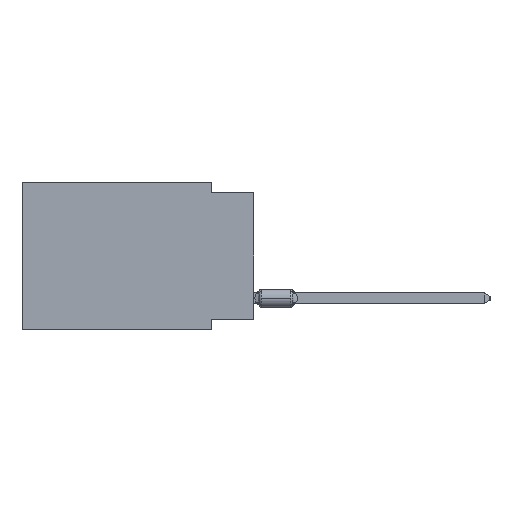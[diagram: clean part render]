
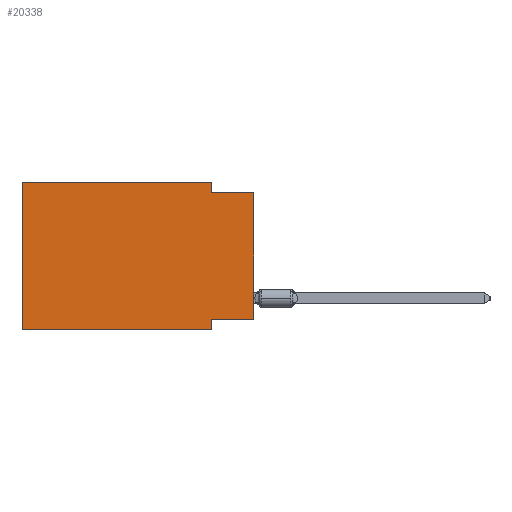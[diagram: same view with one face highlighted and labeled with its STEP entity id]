
A CAD part, left-side view. The second image highlights one B-rep face of the part: STEP entity #20338.
In plain terms, the highlighted planar face has unit normal (-1, 0, 0).
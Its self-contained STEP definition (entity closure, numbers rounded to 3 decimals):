
#49 = LINE ( 'NONE', #8197, #12240 ) ;
#790 = CARTESIAN_POINT ( 'NONE',  ( 0., 13.97, -8.89 ) ) ;
#834 = LINE ( 'NONE', #23825, #12066 ) ;
#2539 = LINE ( 'NONE', #3266, #45087 ) ;
#3266 = CARTESIAN_POINT ( 'NONE',  ( 0., 2.54, 0. ) ) ;
#3526 = DIRECTION ( 'NONE',  ( 0., -1., 0. ) ) ;
#3870 = DIRECTION ( 'NONE',  ( 1., 0., 0. ) ) ;
#4268 = VERTEX_POINT ( 'NONE', #23781 ) ;
#4443 = CARTESIAN_POINT ( 'NONE',  ( 0., 0., 0. ) ) ;
#4548 = CARTESIAN_POINT ( 'NONE',  ( 0., 13.97, 0. ) ) ;
#5168 = VECTOR ( 'NONE', #35991, 1000. ) ;
#5442 = VECTOR ( 'NONE', #29792, 1000. ) ;
#5558 = VERTEX_POINT ( 'NONE', #790 ) ;
#5890 = EDGE_CURVE ( 'NONE', #25024, #8343, #9125, .T. ) ;
#7907 = ORIENTED_EDGE ( 'NONE', *, *, #28779, .F. ) ;
#8197 = CARTESIAN_POINT ( 'NONE',  ( 0., 0., -0.635 ) ) ;
#8343 = VERTEX_POINT ( 'NONE', #45645 ) ;
#8501 = CARTESIAN_POINT ( 'NONE',  ( 0., 2.54, -8.89 ) ) ;
#8968 = EDGE_CURVE ( 'NONE', #5558, #36443, #24704, .T. ) ;
#9125 = LINE ( 'NONE', #4443, #29745 ) ;
#11850 = VECTOR ( 'NONE', #47788, 1000. ) ;
#12066 = VECTOR ( 'NONE', #30796, 1000. ) ;
#12240 = VECTOR ( 'NONE', #3526, 1000. ) ;
#13542 = CARTESIAN_POINT ( 'NONE',  ( 0., 13.97, -8.89 ) ) ;
#14659 = CARTESIAN_POINT ( 'NONE',  ( 0., 2.54, -8.89 ) ) ;
#14978 = PLANE ( 'NONE',  #37952 ) ;
#16639 = CARTESIAN_POINT ( 'NONE',  ( 0., 0., -8.255 ) ) ;
#18688 = CARTESIAN_POINT ( 'NONE',  ( 0., 2.54, 0. ) ) ;
#18935 = DIRECTION ( 'NONE',  ( 0., 0., -1. ) ) ;
#19022 = ORIENTED_EDGE ( 'NONE', *, *, #35650, .F. ) ;
#19498 = DIRECTION ( 'NONE',  ( 0., 0., 1. ) ) ;
#19514 = ORIENTED_EDGE ( 'NONE', *, *, #35379, .F. ) ;
#20338 = ADVANCED_FACE ( 'NONE', ( #48981 ), #14978, .F. ) ;
#23781 = CARTESIAN_POINT ( 'NONE',  ( 0., 2.54, -0.635 ) ) ;
#23825 = CARTESIAN_POINT ( 'NONE',  ( 0., 0., -8.255 ) ) ;
#23869 = CARTESIAN_POINT ( 'NONE',  ( 0., 13.97, 0. ) ) ;
#24704 = LINE ( 'NONE', #13542, #11850 ) ;
#24728 = VERTEX_POINT ( 'NONE', #29064 ) ;
#25024 = VERTEX_POINT ( 'NONE', #16639 ) ;
#25816 = VERTEX_POINT ( 'NONE', #18688 ) ;
#28062 = CARTESIAN_POINT ( 'NONE',  ( 0., 13.97, 0. ) ) ;
#28558 = EDGE_LOOP ( 'NONE', ( #44202, #19022, #40710, #47081, #19514, #42012, #7907, #32492 ) ) ;
#28779 = EDGE_CURVE ( 'NONE', #24728, #36443, #48660, .T. ) ;
#29064 = CARTESIAN_POINT ( 'NONE',  ( 0., 2.54, -8.255 ) ) ;
#29745 = VECTOR ( 'NONE', #19498, 1000. ) ;
#29792 = DIRECTION ( 'NONE',  ( 0., 0., -1. ) ) ;
#30796 = DIRECTION ( 'NONE',  ( 0., 1., 0. ) ) ;
#32137 = EDGE_CURVE ( 'NONE', #25024, #24728, #834, .T. ) ;
#32492 = ORIENTED_EDGE ( 'NONE', *, *, #32137, .F. ) ;
#33137 = EDGE_CURVE ( 'NONE', #37567, #25816, #46725, .T. ) ;
#35379 = EDGE_CURVE ( 'NONE', #5558, #37567, #42989, .T. ) ;
#35650 = EDGE_CURVE ( 'NONE', #4268, #8343, #49, .T. ) ;
#35931 = VECTOR ( 'NONE', #39516, 1000. ) ;
#35991 = DIRECTION ( 'NONE',  ( 0., 0., 1. ) ) ;
#36443 = VERTEX_POINT ( 'NONE', #8501 ) ;
#37567 = VERTEX_POINT ( 'NONE', #4548 ) ;
#37824 = CARTESIAN_POINT ( 'NONE',  ( 0., 13.97, 0. ) ) ;
#37952 = AXIS2_PLACEMENT_3D ( 'NONE', #37824, #3870, #18935 ) ;
#39516 = DIRECTION ( 'NONE',  ( 0., -1., 0. ) ) ;
#39538 = EDGE_CURVE ( 'NONE', #25816, #4268, #2539, .T. ) ;
#40710 = ORIENTED_EDGE ( 'NONE', *, *, #39538, .F. ) ;
#40712 = DIRECTION ( 'NONE',  ( 0., 0., -1. ) ) ;
#42012 = ORIENTED_EDGE ( 'NONE', *, *, #8968, .T. ) ;
#42989 = LINE ( 'NONE', #28062, #5168 ) ;
#44202 = ORIENTED_EDGE ( 'NONE', *, *, #5890, .T. ) ;
#45087 = VECTOR ( 'NONE', #40712, 1000. ) ;
#45645 = CARTESIAN_POINT ( 'NONE',  ( 0., 0., -0.635 ) ) ;
#46725 = LINE ( 'NONE', #23869, #35931 ) ;
#47081 = ORIENTED_EDGE ( 'NONE', *, *, #33137, .F. ) ;
#47788 = DIRECTION ( 'NONE',  ( 0., -1., 0. ) ) ;
#48660 = LINE ( 'NONE', #14659, #5442 ) ;
#48981 = FACE_OUTER_BOUND ( 'NONE', #28558, .T. ) ;
